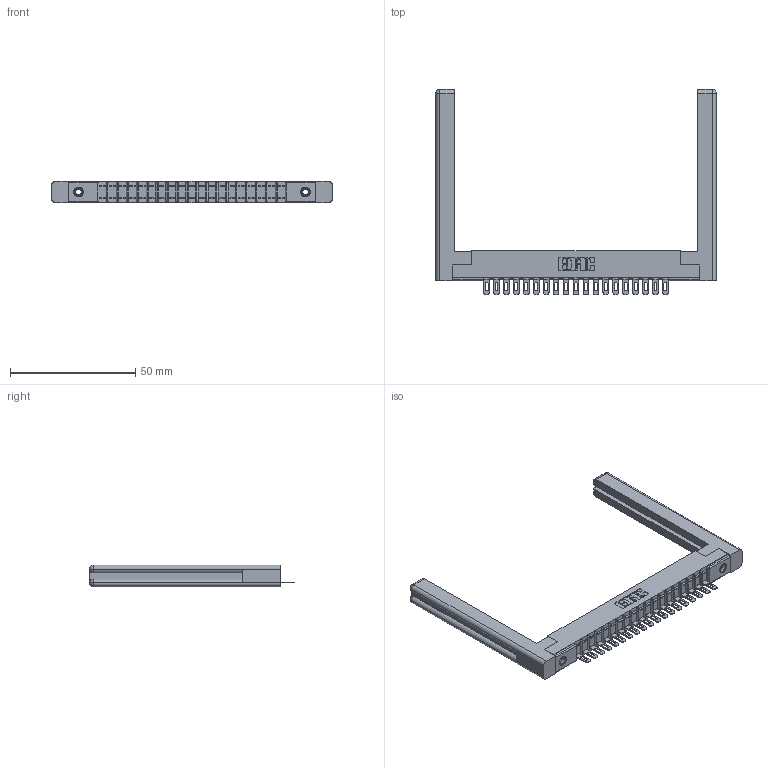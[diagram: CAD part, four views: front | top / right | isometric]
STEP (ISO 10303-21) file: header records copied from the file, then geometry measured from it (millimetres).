
FILE_DESCRIPTION (( 'STEP AP203' ), '1' );
FILE_NAME ('357-019-401-158.STEP', '2020-10-01T02:15:54', ( '' ), ( '' ), 'SwSTEP 2.0', 'SolidWorks 2020', '' );
FILE_SCHEMA (( 'CONFIG_CONTROL_DESIGN' ));
Length unit declared in the file: inch
Products named in the file (5): 345-250-001_345-250-001-102; 307 Part_.156 Dia Mounting Holes; 307-220-058; 357-019-401-158; 307-290-002_501
Assembly tree (24 placements, depth 2):
  357-019-401-158
    307 Part_.156 Dia Mounting Holes
    307-290-002_501  x19
    307-220-058  x2
    345-250-001_345-250-001-102  x2
Bounding box: 111.91 x 81.74 x 8.71 mm (x, y, z)
Volume: 15081.6 mm3; surface area: 18450.6 mm2
Topology: 24 solids, 24 shells, 1724 faces, 5199 edges, 3398 vertices
Faces by surface type: plane 990, cylinder 670, sphere 40, torus 12, cone 12
Entity records: 22551 total; most frequent: CARTESIAN_POINT 3807, ORIENTED_EDGE 3736, DIRECTION 3674, EDGE_CURVE 1868, LINE 1412, VECTOR 1412, VERTEX_POINT 1210, AXIS2_PLACEMENT_3D 1131
